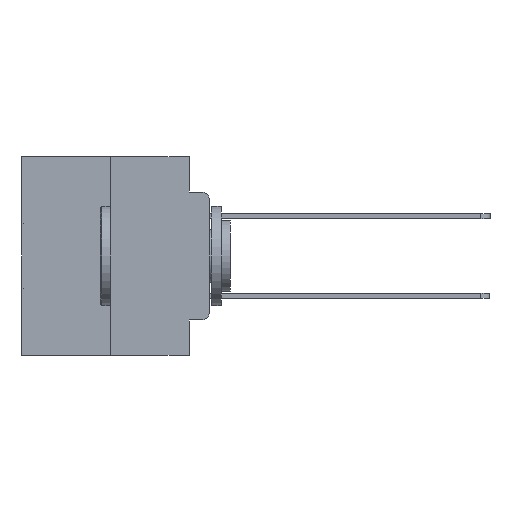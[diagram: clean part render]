
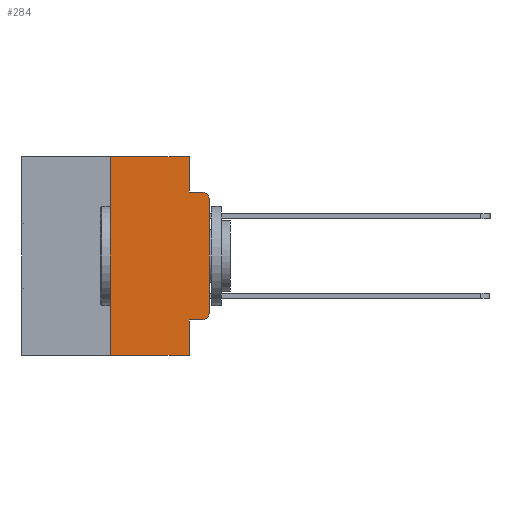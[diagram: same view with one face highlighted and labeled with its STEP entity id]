
A CAD part, left-side view. The second image highlights one B-rep face of the part: STEP entity #284.
In plain terms, the highlighted planar face has unit normal (-1, 0, 0).
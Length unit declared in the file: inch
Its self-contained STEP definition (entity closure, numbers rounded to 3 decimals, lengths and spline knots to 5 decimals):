
#284 = ADVANCED_FACE ( 'NONE', ( #8711 ), #29272, .F. ) ;
#608 = LINE ( 'NONE', #24694, #13004 ) ;
#1125 = CARTESIAN_POINT ( 'NONE',  ( 0., 0.02, -0.4115 ) ) ;
#1464 = DIRECTION ( 'NONE',  ( 0., -1., 0. ) ) ;
#1798 = DIRECTION ( 'NONE',  ( 0., 0., 1. ) ) ;
#2335 = DIRECTION ( 'NONE',  ( 0., 0., -1. ) ) ;
#2384 = VERTEX_POINT ( 'NONE', #25585 ) ;
#2462 = AXIS2_PLACEMENT_3D ( 'NONE', #5318, #22514, #7823 ) ;
#2520 = LINE ( 'NONE', #23976, #21400 ) ;
#3277 = ORIENTED_EDGE ( 'NONE', *, *, #4069, .T. ) ;
#3352 = CARTESIAN_POINT ( 'NONE',  ( 0., 0.02, -0.1085 ) ) ;
#3467 = CARTESIAN_POINT ( 'NONE',  ( 0., 0.051, 0. ) ) ;
#4069 = EDGE_CURVE ( 'NONE', #9811, #16523, #8916, .T. ) ;
#4076 = VERTEX_POINT ( 'NONE', #18080 ) ;
#4328 = CARTESIAN_POINT ( 'NONE',  ( 0., 0., -0.1085 ) ) ;
#4376 = CARTESIAN_POINT ( 'NONE',  ( 0., 0.051, -0.0885 ) ) ;
#5250 = ORIENTED_EDGE ( 'NONE', *, *, #11888, .T. ) ;
#5318 = CARTESIAN_POINT ( 'NONE',  ( 0., 0.02, -0.3915 ) ) ;
#5892 = DIRECTION ( 'NONE',  ( 0., 0., -1. ) ) ;
#6258 = VERTEX_POINT ( 'NONE', #28608 ) ;
#6316 = CARTESIAN_POINT ( 'NONE',  ( 0., 0.051, -0.5 ) ) ;
#7379 = CARTESIAN_POINT ( 'NONE',  ( 0., 0.051, 0. ) ) ;
#7823 = DIRECTION ( 'NONE',  ( 0., 0., -1. ) ) ;
#8033 = EDGE_CURVE ( 'NONE', #6258, #23524, #2520, .T. ) ;
#8711 = FACE_OUTER_BOUND ( 'NONE', #24706, .T. ) ;
#8916 = CIRCLE ( 'NONE', #23506, 0.02 ) ;
#9205 = LINE ( 'NONE', #21205, #21509 ) ;
#9227 = CARTESIAN_POINT ( 'NONE',  ( 0., 0.25, 0. ) ) ;
#9645 = EDGE_CURVE ( 'NONE', #29261, #18641, #12801, .T. ) ;
#9811 = VERTEX_POINT ( 'NONE', #4328 ) ;
#10062 = LINE ( 'NONE', #30905, #20853 ) ;
#10214 = ORIENTED_EDGE ( 'NONE', *, *, #20138, .T. ) ;
#10260 = VERTEX_POINT ( 'NONE', #1125 ) ;
#11015 = DIRECTION ( 'NONE',  ( 0., -1., 0. ) ) ;
#11153 = CARTESIAN_POINT ( 'NONE',  ( 0., 0.02, -0.0885 ) ) ;
#11845 = DIRECTION ( 'NONE',  ( 1., 0., 0. ) ) ;
#11888 = EDGE_CURVE ( 'NONE', #10260, #2384, #20768, .T. ) ;
#12134 = ORIENTED_EDGE ( 'NONE', *, *, #9645, .F. ) ;
#12314 = EDGE_CURVE ( 'NONE', #2384, #9811, #25671, .T. ) ;
#12801 = LINE ( 'NONE', #3467, #26597 ) ;
#12873 = VERTEX_POINT ( 'NONE', #6316 ) ;
#12896 = ORIENTED_EDGE ( 'NONE', *, *, #14093, .F. ) ;
#12919 = EDGE_CURVE ( 'NONE', #18641, #16523, #9205, .T. ) ;
#13004 = VECTOR ( 'NONE', #27118, 39.37008 ) ;
#13243 = EDGE_CURVE ( 'NONE', #6258, #12873, #608, .T. ) ;
#13827 = DIRECTION ( 'NONE',  ( 0., -1., 0. ) ) ;
#14093 = EDGE_CURVE ( 'NONE', #23524, #29261, #17214, .T. ) ;
#14120 = VECTOR ( 'NONE', #2335, 39.37008 ) ;
#14309 = CARTESIAN_POINT ( 'NONE',  ( 0., 0., 0. ) ) ;
#14468 = ORIENTED_EDGE ( 'NONE', *, *, #8033, .F. ) ;
#14829 = ORIENTED_EDGE ( 'NONE', *, *, #12314, .T. ) ;
#14893 = LINE ( 'NONE', #7379, #14120 ) ;
#15221 = ORIENTED_EDGE ( 'NONE', *, *, #13243, .T. ) ;
#16360 = ORIENTED_EDGE ( 'NONE', *, *, #12919, .F. ) ;
#16523 = VERTEX_POINT ( 'NONE', #11153 ) ;
#17214 = LINE ( 'NONE', #28154, #23749 ) ;
#18080 = CARTESIAN_POINT ( 'NONE',  ( 0., 0.051, -0.4115 ) ) ;
#18641 = VERTEX_POINT ( 'NONE', #4376 ) ;
#19175 = VECTOR ( 'NONE', #19244, 39.37008 ) ;
#19244 = DIRECTION ( 'NONE',  ( 0., 0., 1. ) ) ;
#20138 = EDGE_CURVE ( 'NONE', #4076, #10260, #10062, .T. ) ;
#20437 = DIRECTION ( 'NONE',  ( 0., 0., -1. ) ) ;
#20581 = DIRECTION ( 'NONE',  ( -1., 0., 0. ) ) ;
#20697 = DIRECTION ( 'NONE',  ( 0., 0., -1. ) ) ;
#20768 = CIRCLE ( 'NONE', #2462, 0.02 ) ;
#20853 = VECTOR ( 'NONE', #13827, 39.37008 ) ;
#21205 = CARTESIAN_POINT ( 'NONE',  ( 0., 0.051, -0.0885 ) ) ;
#21400 = VECTOR ( 'NONE', #1798, 39.37008 ) ;
#21509 = VECTOR ( 'NONE', #1464, 39.37008 ) ;
#22514 = DIRECTION ( 'NONE',  ( -1., 0., 0. ) ) ;
#23506 = AXIS2_PLACEMENT_3D ( 'NONE', #3352, #20581, #5892 ) ;
#23524 = VERTEX_POINT ( 'NONE', #9227 ) ;
#23749 = VECTOR ( 'NONE', #11015, 39.37008 ) ;
#23976 = CARTESIAN_POINT ( 'NONE',  ( 0., 0.25, 0. ) ) ;
#24694 = CARTESIAN_POINT ( 'NONE',  ( 0., 0.473, -0.5 ) ) ;
#24706 = EDGE_LOOP ( 'NONE', ( #14829, #3277, #16360, #12134, #12896, #14468, #15221, #28983, #10214, #5250 ) ) ;
#25585 = CARTESIAN_POINT ( 'NONE',  ( 0., 0., -0.3915 ) ) ;
#25671 = LINE ( 'NONE', #14309, #19175 ) ;
#26597 = VECTOR ( 'NONE', #20697, 39.37008 ) ;
#27118 = DIRECTION ( 'NONE',  ( 0., -1., 0. ) ) ;
#28154 = CARTESIAN_POINT ( 'NONE',  ( 0., 0.473, 0. ) ) ;
#28284 = EDGE_CURVE ( 'NONE', #4076, #12873, #14893, .T. ) ;
#28440 = CARTESIAN_POINT ( 'NONE',  ( 0., 0.051, 0. ) ) ;
#28608 = CARTESIAN_POINT ( 'NONE',  ( 0., 0.25, -0.5 ) ) ;
#28983 = ORIENTED_EDGE ( 'NONE', *, *, #28284, .F. ) ;
#29126 = AXIS2_PLACEMENT_3D ( 'NONE', #29426, #11845, #20437 ) ;
#29261 = VERTEX_POINT ( 'NONE', #28440 ) ;
#29272 = PLANE ( 'NONE',  #29126 ) ;
#29426 = CARTESIAN_POINT ( 'NONE',  ( 0., 0.473, 0. ) ) ;
#30905 = CARTESIAN_POINT ( 'NONE',  ( 0., 0.051, -0.4115 ) ) ;
